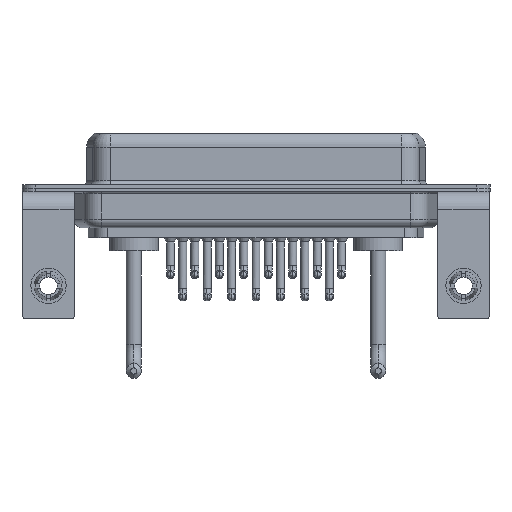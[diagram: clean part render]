
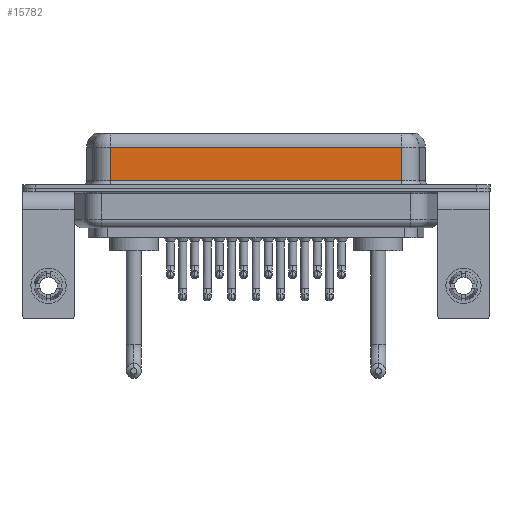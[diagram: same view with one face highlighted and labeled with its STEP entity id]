
A CAD part, front view. The second image highlights one B-rep face of the part: STEP entity #15782.
In plain terms, the highlighted planar face has unit normal (0, -1, 0).
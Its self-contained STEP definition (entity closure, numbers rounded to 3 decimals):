
#1085 = VERTEX_POINT ( 'NONE', #13360 ) ;
#1870 = LINE ( 'NONE', #19858, #4943 ) ;
#2925 = EDGE_CURVE ( 'NONE', #4336, #1085, #5166, .T. ) ;
#3119 = FACE_OUTER_BOUND ( 'NONE', #9450, .T. ) ;
#4107 = VECTOR ( 'NONE', #20758, 1000. ) ;
#4154 = VERTEX_POINT ( 'NONE', #22706 ) ;
#4336 = VERTEX_POINT ( 'NONE', #16122 ) ;
#4341 = VECTOR ( 'NONE', #7146, 1000. ) ;
#4344 = ORIENTED_EDGE ( 'NONE', *, *, #2925, .T. ) ;
#4872 = DIRECTION ( 'NONE',  ( 0., 1., 0. ) ) ;
#4943 = VECTOR ( 'NONE', #17642, 1000. ) ;
#5166 = LINE ( 'NONE', #22810, #9328 ) ;
#7146 = DIRECTION ( 'NONE',  ( 0., 0., -1. ) ) ;
#7525 = EDGE_CURVE ( 'NONE', #10857, #4336, #1870, .T. ) ;
#8478 = DIRECTION ( 'NONE',  ( 1., 0., 0. ) ) ;
#9328 = VECTOR ( 'NONE', #8478, 1000. ) ;
#9450 = EDGE_LOOP ( 'NONE', ( #12361, #9832, #15553, #4344 ) ) ;
#9832 = ORIENTED_EDGE ( 'NONE', *, *, #19395, .T. ) ;
#10410 = AXIS2_PLACEMENT_3D ( 'NONE', #13848, #4872, #12066 ) ;
#10688 = EDGE_CURVE ( 'NONE', #4154, #1085, #17503, .T. ) ;
#10857 = VERTEX_POINT ( 'NONE', #19967 ) ;
#12066 = DIRECTION ( 'NONE',  ( 0., 0., 1. ) ) ;
#12361 = ORIENTED_EDGE ( 'NONE', *, *, #10688, .F. ) ;
#13360 = CARTESIAN_POINT ( 'NONE',  ( 40.037, -3.95, 0.9 ) ) ;
#13628 = CARTESIAN_POINT ( 'NONE',  ( 40.037, -3.95, 4.65 ) ) ;
#13848 = CARTESIAN_POINT ( 'NONE',  ( 40.037, -3.95, 6.4 ) ) ;
#15553 = ORIENTED_EDGE ( 'NONE', *, *, #7525, .T. ) ;
#15782 = ADVANCED_FACE ( 'NONE', ( #3119 ), #22960, .F. ) ;
#16122 = CARTESIAN_POINT ( 'NONE',  ( 7.013, -3.95, 0.9 ) ) ;
#17503 = LINE ( 'NONE', #21133, #4341 ) ;
#17642 = DIRECTION ( 'NONE',  ( 0., 0., -1. ) ) ;
#19395 = EDGE_CURVE ( 'NONE', #4154, #10857, #22404, .T. ) ;
#19858 = CARTESIAN_POINT ( 'NONE',  ( 7.013, -3.95, 6.4 ) ) ;
#19967 = CARTESIAN_POINT ( 'NONE',  ( 7.013, -3.95, 4.65 ) ) ;
#20758 = DIRECTION ( 'NONE',  ( -1., 0., 0. ) ) ;
#21133 = CARTESIAN_POINT ( 'NONE',  ( 40.037, -3.95, 6.4 ) ) ;
#22404 = LINE ( 'NONE', #13628, #4107 ) ;
#22706 = CARTESIAN_POINT ( 'NONE',  ( 40.037, -3.95, 4.65 ) ) ;
#22810 = CARTESIAN_POINT ( 'NONE',  ( 40.037, -3.95, 0.9 ) ) ;
#22960 = PLANE ( 'NONE',  #10410 ) ;
